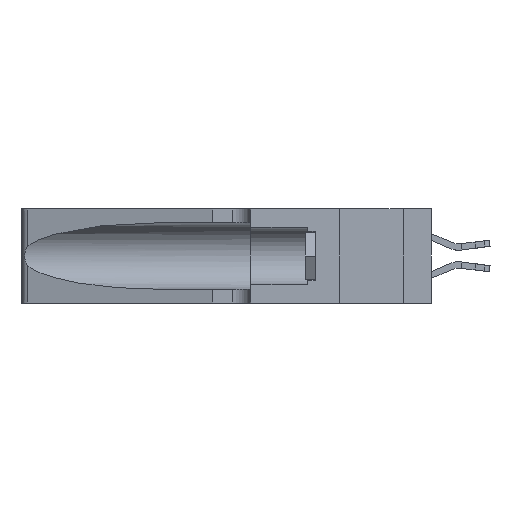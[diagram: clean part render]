
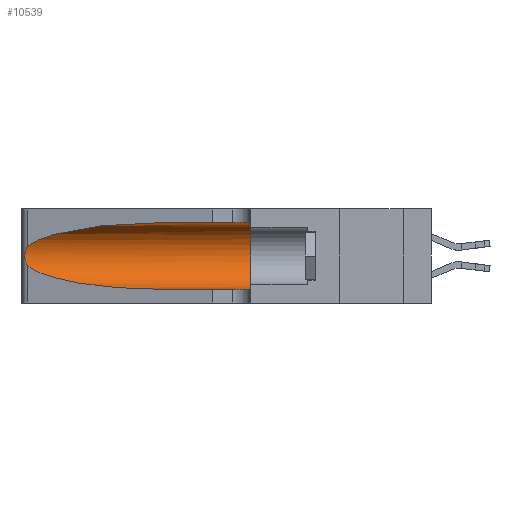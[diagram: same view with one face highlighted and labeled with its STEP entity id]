
A CAD part, left-side view. The second image highlights one B-rep face of the part: STEP entity #10539.
In plain terms, the highlighted cylindrical face has radius 3.308 mm (diameter 6.617 mm), a partial arc.
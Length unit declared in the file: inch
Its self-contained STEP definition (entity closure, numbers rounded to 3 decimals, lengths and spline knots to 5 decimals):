
#662 = CARTESIAN_POINT ( 'NONE',  ( 0.25555, 1.22994, 0.2215 ) ) ;
#1718 = AXIS2_PLACEMENT_3D ( 'NONE', #16599, #27097, #6003 ) ;
#1879 = B_SPLINE_CURVE_WITH_KNOTS ( 'NONE', 3,
 ( #11310, #662, #29424, #13808, #31942, #16430, #21884, #16779, #14163, #11657, #32169, #8802, #22003, #24151 ),
 .UNSPECIFIED., .F., .F.,
 ( 4, 2, 2, 2, 2, 2, 4 ),
 ( 0., 0.00027, 0.00053, 0.00107, 0.0016, 0.00187, 0.00214 ),
 .UNSPECIFIED. ) ;
#3719 = VERTEX_POINT ( 'NONE', #5996 ) ;
#3975 = ORIENTED_EDGE ( 'NONE', *, *, #20051, .T. ) ;
#4455 = VECTOR ( 'NONE', #7280, 39.37008 ) ;
#4719 = CARTESIAN_POINT ( 'NONE',  ( 0.25487, 1.22718, 0.14631 ) ) ;
#5051 =( BOUNDED_CURVE ( )  B_SPLINE_CURVE ( 3, ( #31679, #28964, #21606, #13343 ),
 .UNSPECIFIED., .F., .T. ) 
 B_SPLINE_CURVE_WITH_KNOTS ( ( 4, 4 ),
 ( 1.5708, 2.84003 ),
 .UNSPECIFIED. ) 
 CURVE ( )  GEOMETRIC_REPRESENTATION_ITEM ( )  RATIONAL_B_SPLINE_CURVE ( ( 1., 0.87, 0.87, 1. ) ) 
 REPRESENTATION_ITEM ( '' )  );
#5996 = CARTESIAN_POINT ( 'NONE',  ( 0.1305, 0.72297, 0.05475 ) ) ;
#6003 = DIRECTION ( 'NONE',  ( 0., 0., 1. ) ) ;
#7108 = CARTESIAN_POINT ( 'NONE',  ( 0.1305, 0.72297, 0.05475 ) ) ;
#7280 = DIRECTION ( 'NONE',  ( 0., -1., 0. ) ) ;
#7352 = CARTESIAN_POINT ( 'NONE',  ( 0.1305, 0.35, 0.31525 ) ) ;
#8802 = CARTESIAN_POINT ( 'NONE',  ( 0.25639, 1.23186, 0.15144 ) ) ;
#8936 = CYLINDRICAL_SURFACE ( 'NONE', #18063, 0.13025 ) ;
#9622 =( BOUNDED_CURVE ( )  B_SPLINE_CURVE ( 3, ( #4719, #27968, #22912, #7108 ),
 .UNSPECIFIED., .F., .F. ) 
 B_SPLINE_CURVE_WITH_KNOTS ( ( 4, 4 ),
 ( 3.44316, 4.71239 ),
 .UNSPECIFIED. ) 
 CURVE ( )  GEOMETRIC_REPRESENTATION_ITEM ( )  RATIONAL_B_SPLINE_CURVE ( ( 1., 0.87, 0.87, 1. ) ) 
 REPRESENTATION_ITEM ( '' )  );
#10346 = ORIENTED_EDGE ( 'NONE', *, *, #31329, .F. ) ;
#10539 = ADVANCED_FACE ( 'NONE', ( #15099 ), #8936, .F. ) ;
#11310 = CARTESIAN_POINT ( 'NONE',  ( 0.25487, 1.22718, 0.22369 ) ) ;
#11657 = CARTESIAN_POINT ( 'NONE',  ( 0.25856, 1.23593, 0.16098 ) ) ;
#12878 = DIRECTION ( 'NONE',  ( 0., 0., -1. ) ) ;
#13343 = CARTESIAN_POINT ( 'NONE',  ( 0.25487, 1.22718, 0.22369 ) ) ;
#13808 = CARTESIAN_POINT ( 'NONE',  ( 0.25787, 1.23484, 0.2124 ) ) ;
#14163 = CARTESIAN_POINT ( 'NONE',  ( 0.26017, 1.23833, 0.17102 ) ) ;
#14475 = VERTEX_POINT ( 'NONE', #7352 ) ;
#14702 = VERTEX_POINT ( 'NONE', #14916 ) ;
#14916 = CARTESIAN_POINT ( 'NONE',  ( 0.25487, 1.22718, 0.14631 ) ) ;
#15099 = FACE_OUTER_BOUND ( 'NONE', #27003, .T. ) ;
#16259 = EDGE_CURVE ( 'NONE', #3719, #30563, #22362, .T. ) ;
#16430 = CARTESIAN_POINT ( 'NONE',  ( 0.26018, 1.23835, 0.19895 ) ) ;
#16599 = CARTESIAN_POINT ( 'NONE',  ( 0.1305, 0.35, 0.185 ) ) ;
#16779 = CARTESIAN_POINT ( 'NONE',  ( 0.26075, 1.23896, 0.178 ) ) ;
#17831 = CARTESIAN_POINT ( 'NONE',  ( 0.1305, 1.61858, 0.05475 ) ) ;
#18063 = AXIS2_PLACEMENT_3D ( 'NONE', #33459, #22901, #12878 ) ;
#19076 = CARTESIAN_POINT ( 'NONE',  ( 0.25487, 1.22718, 0.22369 ) ) ;
#20051 = EDGE_CURVE ( 'NONE', #14702, #3719, #9622, .T. ) ;
#20599 = VECTOR ( 'NONE', #27678, 39.37008 ) ;
#21606 = CARTESIAN_POINT ( 'NONE',  ( 0.2373, 1.15595, 0.28018 ) ) ;
#21884 = CARTESIAN_POINT ( 'NONE',  ( 0.26075, 1.23896, 0.19203 ) ) ;
#22003 = CARTESIAN_POINT ( 'NONE',  ( 0.25555, 1.22993, 0.14849 ) ) ;
#22362 = LINE ( 'NONE', #17831, #4455 ) ;
#22901 = DIRECTION ( 'NONE',  ( 0., -1., 0. ) ) ;
#22912 = CARTESIAN_POINT ( 'NONE',  ( 0.18966, 0.96281, 0.05475 ) ) ;
#23157 = ORIENTED_EDGE ( 'NONE', *, *, #26723, .T. ) ;
#23752 = EDGE_CURVE ( 'NONE', #14475, #30563, #27681, .T. ) ;
#23939 = VERTEX_POINT ( 'NONE', #27411 ) ;
#24151 = CARTESIAN_POINT ( 'NONE',  ( 0.25487, 1.22718, 0.14631 ) ) ;
#26148 = EDGE_CURVE ( 'NONE', #29236, #14702, #1879, .T. ) ;
#26723 = EDGE_CURVE ( 'NONE', #23939, #29236, #5051, .T. ) ;
#27003 = EDGE_LOOP ( 'NONE', ( #23157, #32352, #3975, #32108, #31526, #10346 ) ) ;
#27097 = DIRECTION ( 'NONE',  ( 0., 1., 0. ) ) ;
#27411 = CARTESIAN_POINT ( 'NONE',  ( 0.1305, 0.72297, 0.31525 ) ) ;
#27597 = CARTESIAN_POINT ( 'NONE',  ( 0.1305, 0.35, 0.05475 ) ) ;
#27678 = DIRECTION ( 'NONE',  ( 0., -1., 0. ) ) ;
#27681 = CIRCLE ( 'NONE', #1718, 0.13025 ) ;
#27968 = CARTESIAN_POINT ( 'NONE',  ( 0.2373, 1.15595, 0.08982 ) ) ;
#28964 = CARTESIAN_POINT ( 'NONE',  ( 0.18966, 0.96281, 0.31525 ) ) ;
#29236 = VERTEX_POINT ( 'NONE', #19076 ) ;
#29424 = CARTESIAN_POINT ( 'NONE',  ( 0.25639, 1.23184, 0.21858 ) ) ;
#30169 = CARTESIAN_POINT ( 'NONE',  ( 0.1305, 1.61858, 0.31525 ) ) ;
#30563 = VERTEX_POINT ( 'NONE', #27597 ) ;
#31329 = EDGE_CURVE ( 'NONE', #23939, #14475, #32744, .T. ) ;
#31526 = ORIENTED_EDGE ( 'NONE', *, *, #23752, .F. ) ;
#31679 = CARTESIAN_POINT ( 'NONE',  ( 0.1305, 0.72297, 0.31525 ) ) ;
#31942 = CARTESIAN_POINT ( 'NONE',  ( 0.25854, 1.2359, 0.20912 ) ) ;
#32108 = ORIENTED_EDGE ( 'NONE', *, *, #16259, .T. ) ;
#32169 = CARTESIAN_POINT ( 'NONE',  ( 0.25789, 1.23486, 0.15765 ) ) ;
#32352 = ORIENTED_EDGE ( 'NONE', *, *, #26148, .T. ) ;
#32744 = LINE ( 'NONE', #30169, #20599 ) ;
#33459 = CARTESIAN_POINT ( 'NONE',  ( 0.1305, 1.61858, 0.185 ) ) ;
